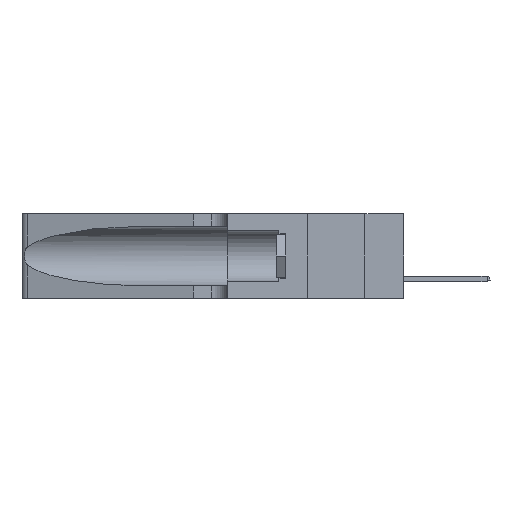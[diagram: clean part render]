
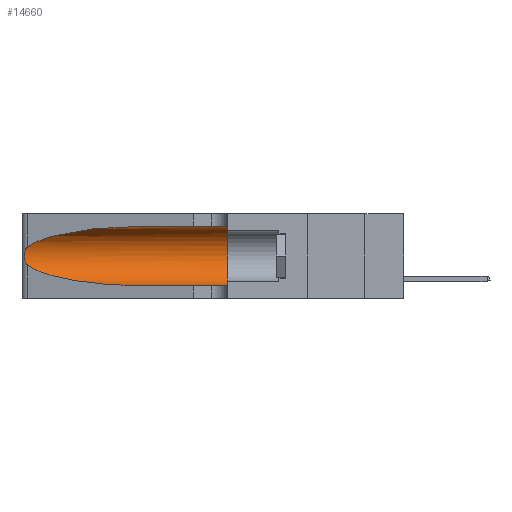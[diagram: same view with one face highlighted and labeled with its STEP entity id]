
A CAD part, left-side view. The second image highlights one B-rep face of the part: STEP entity #14660.
In plain terms, the highlighted cylindrical face has radius 3.308 mm (diameter 6.617 mm), a partial arc.
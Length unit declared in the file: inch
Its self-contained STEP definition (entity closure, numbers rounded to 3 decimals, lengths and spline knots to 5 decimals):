
#482 = CARTESIAN_POINT ( 'NONE',  ( 0.2373, 1.15595, 0.08982 ) ) ;
#971 = VERTEX_POINT ( 'NONE', #21411 ) ;
#1175 = EDGE_CURVE ( 'NONE', #19012, #971, #5435, .T. ) ;
#1267 = CARTESIAN_POINT ( 'NONE',  ( 0.1305, 0.72297, 0.31525 ) ) ;
#1899 = DIRECTION ( 'NONE',  ( 0., 0., -1. ) ) ;
#1918 = CARTESIAN_POINT ( 'NONE',  ( 0.25487, 1.22718, 0.14631 ) ) ;
#2042 = CARTESIAN_POINT ( 'NONE',  ( 0.25789, 1.23486, 0.15765 ) ) ;
#2293 = DIRECTION ( 'NONE',  ( 0., -1., 0. ) ) ;
#2517 = ORIENTED_EDGE ( 'NONE', *, *, #14058, .F. ) ;
#3808 = AXIS2_PLACEMENT_3D ( 'NONE', #10639, #15072, #6200 ) ;
#4010 = CARTESIAN_POINT ( 'NONE',  ( 0.26017, 1.23833, 0.17102 ) ) ;
#4091 = CARTESIAN_POINT ( 'NONE',  ( 0.25555, 1.22993, 0.14849 ) ) ;
#4746 = CYLINDRICAL_SURFACE ( 'NONE', #15035, 0.13025 ) ;
#5435 =( BOUNDED_CURVE ( )  B_SPLINE_CURVE ( 3, ( #1267, #11170, #6500, #5969 ),
 .UNSPECIFIED., .F., .F. ) 
 B_SPLINE_CURVE_WITH_KNOTS ( ( 4, 4 ),
 ( 1.5708, 2.84003 ),
 .UNSPECIFIED. ) 
 CURVE ( )  GEOMETRIC_REPRESENTATION_ITEM ( )  RATIONAL_B_SPLINE_CURVE ( ( 1., 0.87, 0.87, 1. ) ) 
 REPRESENTATION_ITEM ( '' )  );
#5912 = CARTESIAN_POINT ( 'NONE',  ( 0.1305, 0.72297, 0.31525 ) ) ;
#5969 = CARTESIAN_POINT ( 'NONE',  ( 0.25487, 1.22718, 0.22369 ) ) ;
#6122 = FACE_OUTER_BOUND ( 'NONE', #8227, .T. ) ;
#6200 = DIRECTION ( 'NONE',  ( 0., 0., 1. ) ) ;
#6500 = CARTESIAN_POINT ( 'NONE',  ( 0.2373, 1.15595, 0.28018 ) ) ;
#6553 = ORIENTED_EDGE ( 'NONE', *, *, #12758, .F. ) ;
#8128 = B_SPLINE_CURVE_WITH_KNOTS ( 'NONE', 3,
 ( #17519, #11026, #19629, #9322, #21407, #14401, #16171, #14543, #4010, #18094, #2042, #21642, #4091, #19558 ),
 .UNSPECIFIED., .F., .F.,
 ( 4, 2, 2, 2, 2, 2, 4 ),
 ( 0., 0.00027, 0.00053, 0.00107, 0.0016, 0.00187, 0.00214 ),
 .UNSPECIFIED. ) ;
#8135 = CARTESIAN_POINT ( 'NONE',  ( 0.1305, 1.61858, 0.05475 ) ) ;
#8227 = EDGE_LOOP ( 'NONE', ( #14908, #21013, #12641, #13991, #6553, #2517 ) ) ;
#9103 =( BOUNDED_CURVE ( )  B_SPLINE_CURVE ( 3, ( #12648, #482, #16397, #9253 ),
 .UNSPECIFIED., .F., .F. ) 
 B_SPLINE_CURVE_WITH_KNOTS ( ( 4, 4 ),
 ( 3.44316, 4.71239 ),
 .UNSPECIFIED. ) 
 CURVE ( )  GEOMETRIC_REPRESENTATION_ITEM ( )  RATIONAL_B_SPLINE_CURVE ( ( 1., 0.87, 0.87, 1. ) ) 
 REPRESENTATION_ITEM ( '' )  );
#9253 = CARTESIAN_POINT ( 'NONE',  ( 0.1305, 0.72297, 0.05475 ) ) ;
#9322 = CARTESIAN_POINT ( 'NONE',  ( 0.25787, 1.23484, 0.2124 ) ) ;
#10272 = LINE ( 'NONE', #13971, #18802 ) ;
#10639 = CARTESIAN_POINT ( 'NONE',  ( 0.1305, 0.35, 0.185 ) ) ;
#11026 = CARTESIAN_POINT ( 'NONE',  ( 0.25555, 1.22994, 0.2215 ) ) ;
#11170 = CARTESIAN_POINT ( 'NONE',  ( 0.18966, 0.96281, 0.31525 ) ) ;
#11216 = CARTESIAN_POINT ( 'NONE',  ( 0.1305, 0.35, 0.31525 ) ) ;
#11403 = LINE ( 'NONE', #8135, #15532 ) ;
#11494 = CARTESIAN_POINT ( 'NONE',  ( 0.1305, 0.72297, 0.05475 ) ) ;
#12641 = ORIENTED_EDGE ( 'NONE', *, *, #12771, .T. ) ;
#12648 = CARTESIAN_POINT ( 'NONE',  ( 0.25487, 1.22718, 0.14631 ) ) ;
#12708 = VERTEX_POINT ( 'NONE', #20325 ) ;
#12758 = EDGE_CURVE ( 'NONE', #20752, #12708, #15553, .T. ) ;
#12771 = EDGE_CURVE ( 'NONE', #20263, #17304, #9103, .T. ) ;
#13108 = EDGE_CURVE ( 'NONE', #17304, #12708, #11403, .T. ) ;
#13971 = CARTESIAN_POINT ( 'NONE',  ( 0.1305, 1.61858, 0.31525 ) ) ;
#13991 = ORIENTED_EDGE ( 'NONE', *, *, #13108, .T. ) ;
#14058 = EDGE_CURVE ( 'NONE', #19012, #20752, #10272, .T. ) ;
#14401 = CARTESIAN_POINT ( 'NONE',  ( 0.26018, 1.23835, 0.19895 ) ) ;
#14543 = CARTESIAN_POINT ( 'NONE',  ( 0.26075, 1.23896, 0.178 ) ) ;
#14660 = ADVANCED_FACE ( 'NONE', ( #6122 ), #4746, .F. ) ;
#14908 = ORIENTED_EDGE ( 'NONE', *, *, #1175, .T. ) ;
#15035 = AXIS2_PLACEMENT_3D ( 'NONE', #15202, #18745, #1899 ) ;
#15072 = DIRECTION ( 'NONE',  ( 0., 1., 0. ) ) ;
#15202 = CARTESIAN_POINT ( 'NONE',  ( 0.1305, 1.61858, 0.185 ) ) ;
#15532 = VECTOR ( 'NONE', #2293, 39.37008 ) ;
#15553 = CIRCLE ( 'NONE', #3808, 0.13025 ) ;
#16171 = CARTESIAN_POINT ( 'NONE',  ( 0.26075, 1.23896, 0.19203 ) ) ;
#16397 = CARTESIAN_POINT ( 'NONE',  ( 0.18966, 0.96281, 0.05475 ) ) ;
#17304 = VERTEX_POINT ( 'NONE', #11494 ) ;
#17519 = CARTESIAN_POINT ( 'NONE',  ( 0.25487, 1.22718, 0.22369 ) ) ;
#18094 = CARTESIAN_POINT ( 'NONE',  ( 0.25856, 1.23593, 0.16098 ) ) ;
#18745 = DIRECTION ( 'NONE',  ( 0., -1., 0. ) ) ;
#18802 = VECTOR ( 'NONE', #19269, 39.37008 ) ;
#19012 = VERTEX_POINT ( 'NONE', #5912 ) ;
#19269 = DIRECTION ( 'NONE',  ( 0., -1., 0. ) ) ;
#19558 = CARTESIAN_POINT ( 'NONE',  ( 0.25487, 1.22718, 0.14631 ) ) ;
#19629 = CARTESIAN_POINT ( 'NONE',  ( 0.25639, 1.23184, 0.21858 ) ) ;
#20263 = VERTEX_POINT ( 'NONE', #1918 ) ;
#20325 = CARTESIAN_POINT ( 'NONE',  ( 0.1305, 0.35, 0.05475 ) ) ;
#20752 = VERTEX_POINT ( 'NONE', #11216 ) ;
#20886 = EDGE_CURVE ( 'NONE', #971, #20263, #8128, .T. ) ;
#21013 = ORIENTED_EDGE ( 'NONE', *, *, #20886, .T. ) ;
#21407 = CARTESIAN_POINT ( 'NONE',  ( 0.25854, 1.2359, 0.20912 ) ) ;
#21411 = CARTESIAN_POINT ( 'NONE',  ( 0.25487, 1.22718, 0.22369 ) ) ;
#21642 = CARTESIAN_POINT ( 'NONE',  ( 0.25639, 1.23186, 0.15144 ) ) ;
